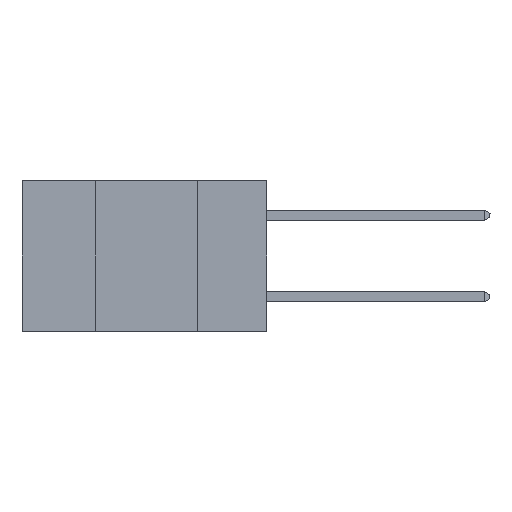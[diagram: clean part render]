
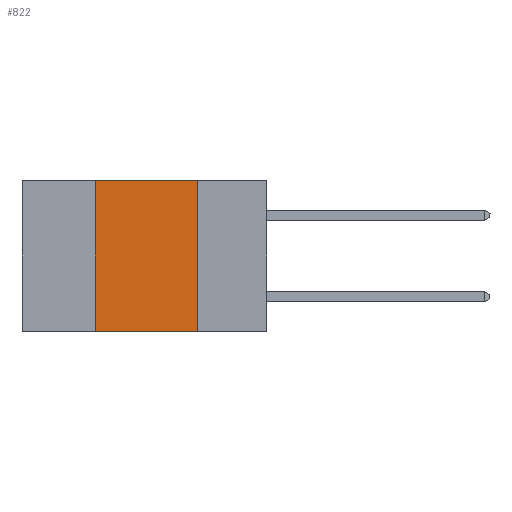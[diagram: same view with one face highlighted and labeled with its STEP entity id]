
A CAD part, left-side view. The second image highlights one B-rep face of the part: STEP entity #822.
In plain terms, the highlighted planar face has unit normal (-1, 0, 0).
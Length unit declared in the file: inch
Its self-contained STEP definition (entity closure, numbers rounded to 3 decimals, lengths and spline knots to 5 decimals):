
#114 = CARTESIAN_POINT ( 'NONE',  ( 0., 0.17, -0.37 ) ) ;
#822 = ADVANCED_FACE ( 'NONE', ( #10763 ), #8359, .F. ) ;
#980 = EDGE_LOOP ( 'NONE', ( #1886, #7134, #6182, #8097 ) ) ;
#989 = EDGE_CURVE ( 'NONE', #10030, #5093, #8903, .T. ) ;
#1361 = DIRECTION ( 'NONE',  ( 0., 0., 1. ) ) ;
#1386 = EDGE_CURVE ( 'NONE', #9582, #10030, #3986, .T. ) ;
#1600 = CARTESIAN_POINT ( 'NONE',  ( 0., 0.42, -0.37 ) ) ;
#1669 = CARTESIAN_POINT ( 'NONE',  ( 0., 0.42, 0. ) ) ;
#1886 = ORIENTED_EDGE ( 'NONE', *, *, #2139, .F. ) ;
#2139 = EDGE_CURVE ( 'NONE', #5093, #2158, #9539, .T. ) ;
#2158 = VERTEX_POINT ( 'NONE', #114 ) ;
#2489 = DIRECTION ( 'NONE',  ( 0., 0., -1. ) ) ;
#2577 = DIRECTION ( 'NONE',  ( 0., 0., -1. ) ) ;
#2912 = CARTESIAN_POINT ( 'NONE',  ( 0., 0.42, 0. ) ) ;
#3307 = EDGE_CURVE ( 'NONE', #9582, #2158, #10937, .T. ) ;
#3890 = DIRECTION ( 'NONE',  ( 0., -1., 0. ) ) ;
#3986 = LINE ( 'NONE', #2912, #10754 ) ;
#4370 = VECTOR ( 'NONE', #2577, 39.37008 ) ;
#4585 = CARTESIAN_POINT ( 'NONE',  ( 0., 0.6, 0. ) ) ;
#4976 = DIRECTION ( 'NONE',  ( 1., 0., 0. ) ) ;
#5093 = VERTEX_POINT ( 'NONE', #9695 ) ;
#6182 = ORIENTED_EDGE ( 'NONE', *, *, #1386, .F. ) ;
#6571 = CARTESIAN_POINT ( 'NONE',  ( 0., 0.6, -0.37 ) ) ;
#6704 = CARTESIAN_POINT ( 'NONE',  ( 0., 0.6, 0. ) ) ;
#7062 = VECTOR ( 'NONE', #8308, 39.37008 ) ;
#7134 = ORIENTED_EDGE ( 'NONE', *, *, #989, .F. ) ;
#7688 = CARTESIAN_POINT ( 'NONE',  ( 0., 0.17, 0. ) ) ;
#8097 = ORIENTED_EDGE ( 'NONE', *, *, #3307, .T. ) ;
#8308 = DIRECTION ( 'NONE',  ( 0., -1., 0. ) ) ;
#8359 = PLANE ( 'NONE',  #9861 ) ;
#8903 = LINE ( 'NONE', #4585, #9564 ) ;
#9539 = LINE ( 'NONE', #7688, #4370 ) ;
#9564 = VECTOR ( 'NONE', #3890, 39.37008 ) ;
#9582 = VERTEX_POINT ( 'NONE', #1600 ) ;
#9695 = CARTESIAN_POINT ( 'NONE',  ( 0., 0.17, 0. ) ) ;
#9861 = AXIS2_PLACEMENT_3D ( 'NONE', #6704, #4976, #2489 ) ;
#10030 = VERTEX_POINT ( 'NONE', #1669 ) ;
#10754 = VECTOR ( 'NONE', #1361, 39.37008 ) ;
#10763 = FACE_OUTER_BOUND ( 'NONE', #980, .T. ) ;
#10937 = LINE ( 'NONE', #6571, #7062 ) ;
